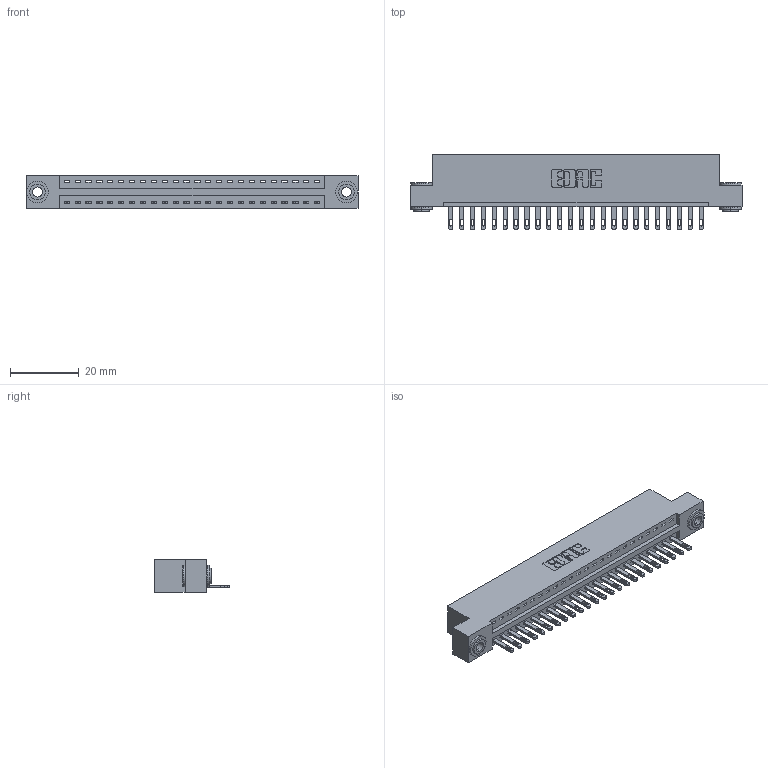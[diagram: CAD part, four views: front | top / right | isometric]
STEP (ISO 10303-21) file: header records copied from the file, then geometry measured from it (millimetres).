
FILE_DESCRIPTION (( 'STEP AP203' ), '1' );
FILE_NAME ('896-024-500-103.STEP', '2021-07-27T17:21:10', ( '' ), ( '' ), 'SwSTEP 2.0', 'SolidWorks 2020', '' );
FILE_SCHEMA (( 'CONFIG_CONTROL_DESIGN' ));
Length unit declared in the file: inch
Products named in the file (4): 896-024-500-103; 345-250-002_345-250-002-102; 345-292-001_345-293-100; 846 Part_Flush Mounting Lugs - 0.156 Dia-TH
Assembly tree (27 placements, depth 2):
  896-024-500-103
    846 Part_Flush Mounting Lugs - 0.156 Dia-TH
    345-292-001_345-293-100  x24
    345-250-002_345-250-002-102  x2
Bounding box: 96.77 x 21.84 x 9.4 mm (x, y, z)
Volume: 9173.6 mm3; surface area: 11546.7 mm2
Topology: 27 solids, 27 shells, 1456 faces, 4437 edges, 2954 vertices
Faces by surface type: plane 902, cylinder 546, cone 8
Entity records: 17898 total; most frequent: CARTESIAN_POINT 3051, ORIENTED_EDGE 3002, DIRECTION 2747, EDGE_CURVE 1501, VECTOR 1245, LINE 1245, VERTEX_POINT 998, AXIS2_PLACEMENT_3D 751
